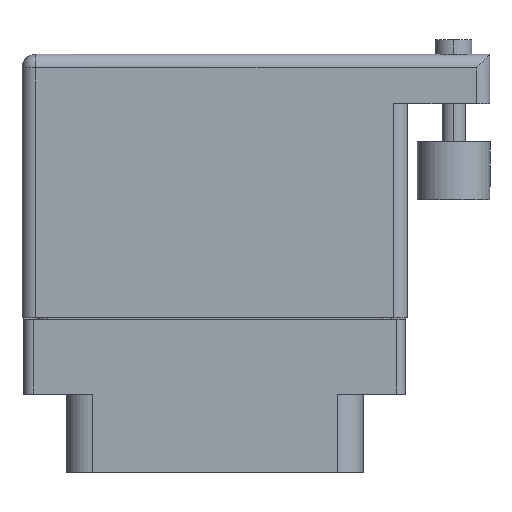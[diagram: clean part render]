
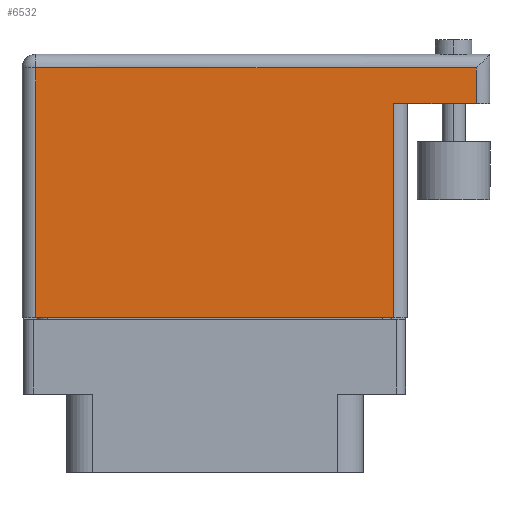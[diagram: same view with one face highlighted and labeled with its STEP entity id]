
A CAD part, front view. The second image highlights one B-rep face of the part: STEP entity #6532.
In plain terms, the highlighted face is planar.
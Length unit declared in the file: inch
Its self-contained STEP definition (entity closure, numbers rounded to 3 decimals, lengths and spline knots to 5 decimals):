
#174 = DIRECTION ( 'NONE',  ( 0., -1., 0. ) ) ;
#3175 = PLANE ( 'NONE',  #26973 ) ;
#3300 = VERTEX_POINT ( 'NONE', #25050 ) ;
#4131 = ORIENTED_EDGE ( 'NONE', *, *, #18437, .T. ) ;
#4291 = DIRECTION ( 'NONE',  ( 0., 1., 0. ) ) ;
#4334 = VECTOR ( 'NONE', #19216, 39.37008 ) ;
#4829 = EDGE_CURVE ( 'NONE', #28817, #16810, #6930, .T. ) ;
#5043 = EDGE_CURVE ( 'NONE', #25837, #6308, #27310, .T. ) ;
#5800 = VERTEX_POINT ( 'NONE', #11395 ) ;
#6308 = VERTEX_POINT ( 'NONE', #12329 ) ;
#6532 = ADVANCED_FACE ( 'NONE', ( #19717 ), #3175, .F. ) ;
#6930 = LINE ( 'NONE', #7401, #4334 ) ;
#7347 = VECTOR ( 'NONE', #174, 39.37008 ) ;
#7401 = CARTESIAN_POINT ( 'NONE',  ( -0.6625, -0.1, 0.3575 ) ) ;
#8998 = DIRECTION ( 'NONE',  ( 0., 1., 0. ) ) ;
#9121 = VECTOR ( 'NONE', #18280, 39.37008 ) ;
#9550 = EDGE_CURVE ( 'NONE', #16810, #6308, #14007, .T. ) ;
#10242 = CARTESIAN_POINT ( 'NONE',  ( -0.6625, 0.806, 0.3575 ) ) ;
#11395 = CARTESIAN_POINT ( 'NONE',  ( 0.8995, 0.759, 0.3575 ) ) ;
#11899 = LINE ( 'NONE', #24521, #27478 ) ;
#12329 = CARTESIAN_POINT ( 'NONE',  ( 0.6155, 0.636, 0.3575 ) ) ;
#12619 = ORIENTED_EDGE ( 'NONE', *, *, #18648, .T. ) ;
#12835 = DIRECTION ( 'NONE',  ( 0., 0., -1. ) ) ;
#14007 = LINE ( 'NONE', #18446, #23647 ) ;
#14180 = ORIENTED_EDGE ( 'NONE', *, *, #9550, .T. ) ;
#14386 = VECTOR ( 'NONE', #4291, 39.37008 ) ;
#14436 = CARTESIAN_POINT ( 'NONE',  ( -0.6155, -0.1, 0.3575 ) ) ;
#15892 = CARTESIAN_POINT ( 'NONE',  ( 0.9465, 0.636, 0.3575 ) ) ;
#16810 = VERTEX_POINT ( 'NONE', #28751 ) ;
#17488 = DIRECTION ( 'NONE',  ( -1., 0., 0. ) ) ;
#17876 = EDGE_LOOP ( 'NONE', ( #22339, #14180, #20716, #12619, #30122, #4131 ) ) ;
#18131 = LINE ( 'NONE', #14436, #7347 ) ;
#18280 = DIRECTION ( 'NONE',  ( -1., 0., 0. ) ) ;
#18437 = EDGE_CURVE ( 'NONE', #3300, #28817, #18131, .T. ) ;
#18446 = CARTESIAN_POINT ( 'NONE',  ( 0.6155, 0.636, 0.3575 ) ) ;
#18648 = EDGE_CURVE ( 'NONE', #25837, #5800, #26985, .T. ) ;
#19216 = DIRECTION ( 'NONE',  ( 1., 0., 0. ) ) ;
#19717 = FACE_OUTER_BOUND ( 'NONE', #17876, .T. ) ;
#20716 = ORIENTED_EDGE ( 'NONE', *, *, #5043, .F. ) ;
#22339 = ORIENTED_EDGE ( 'NONE', *, *, #4829, .T. ) ;
#22376 = DIRECTION ( 'NONE',  ( -1., 0., 0. ) ) ;
#22508 = CARTESIAN_POINT ( 'NONE',  ( -0.6155, -0.1, 0.3575 ) ) ;
#23647 = VECTOR ( 'NONE', #8998, 39.37008 ) ;
#24097 = CARTESIAN_POINT ( 'NONE',  ( 0.8995, 0.636, 0.3575 ) ) ;
#24521 = CARTESIAN_POINT ( 'NONE',  ( -0.6625, 0.759, 0.3575 ) ) ;
#25050 = CARTESIAN_POINT ( 'NONE',  ( -0.6155, 0.759, 0.3575 ) ) ;
#25455 = CARTESIAN_POINT ( 'NONE',  ( 0.8995, 0.806, 0.3575 ) ) ;
#25837 = VERTEX_POINT ( 'NONE', #24097 ) ;
#26973 = AXIS2_PLACEMENT_3D ( 'NONE', #10242, #12835, #22376 ) ;
#26985 = LINE ( 'NONE', #25455, #14386 ) ;
#27156 = EDGE_CURVE ( 'NONE', #5800, #3300, #11899, .T. ) ;
#27310 = LINE ( 'NONE', #15892, #9121 ) ;
#27478 = VECTOR ( 'NONE', #17488, 39.37008 ) ;
#28751 = CARTESIAN_POINT ( 'NONE',  ( 0.6155, -0.1, 0.3575 ) ) ;
#28817 = VERTEX_POINT ( 'NONE', #22508 ) ;
#30122 = ORIENTED_EDGE ( 'NONE', *, *, #27156, .T. ) ;
